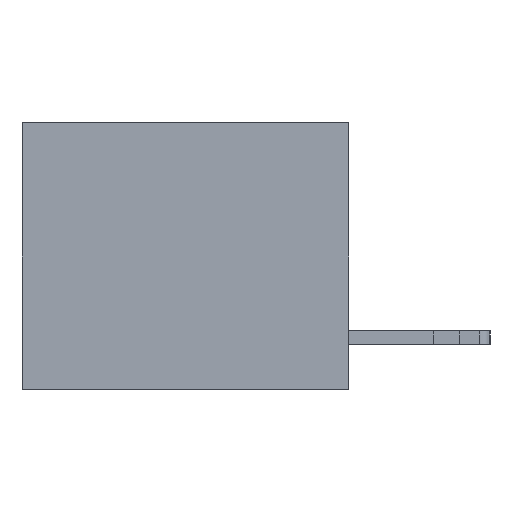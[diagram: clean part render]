
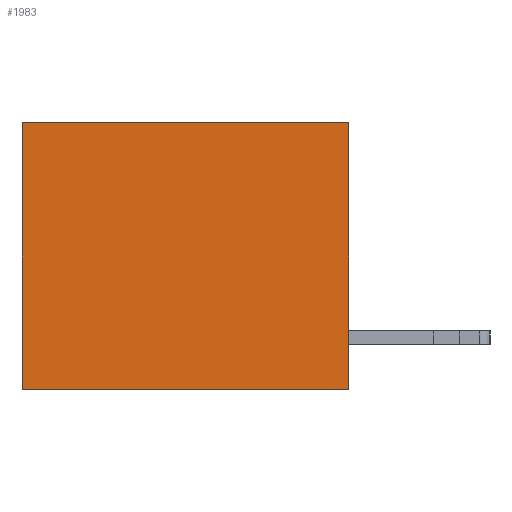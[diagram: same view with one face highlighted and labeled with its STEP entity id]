
A CAD part, left-side view. The second image highlights one B-rep face of the part: STEP entity #1983.
In plain terms, the highlighted planar face has unit normal (-1, 0, 0).
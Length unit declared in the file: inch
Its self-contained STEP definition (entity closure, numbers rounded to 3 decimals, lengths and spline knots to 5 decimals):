
#357 = EDGE_CURVE ( 'NONE', #7541, #11185, #21922, .T. ) ;
#1149 = DIRECTION ( 'NONE',  ( 0., 0., -1. ) ) ;
#1983 = ADVANCED_FACE ( 'NONE', ( #4147 ), #3346, .F. ) ;
#2120 = VECTOR ( 'NONE', #2600, 39.37008 ) ;
#2600 = DIRECTION ( 'NONE',  ( 0., 1., 0. ) ) ;
#2934 = EDGE_CURVE ( 'NONE', #11185, #13010, #17881, .T. ) ;
#3230 = DIRECTION ( 'NONE',  ( 0., 1., 0. ) ) ;
#3346 = PLANE ( 'NONE',  #8879 ) ;
#4147 = FACE_OUTER_BOUND ( 'NONE', #4402, .T. ) ;
#4402 = EDGE_LOOP ( 'NONE', ( #14719, #14878, #11434, #5678 ) ) ;
#4917 = CARTESIAN_POINT ( 'NONE',  ( 0.3165, 0.6, -0.49 ) ) ;
#5678 = ORIENTED_EDGE ( 'NONE', *, *, #357, .T. ) ;
#5765 = EDGE_CURVE ( 'NONE', #7255, #13010, #18853, .T. ) ;
#5997 = EDGE_CURVE ( 'NONE', #7541, #7255, #20634, .T. ) ;
#6631 = CARTESIAN_POINT ( 'NONE',  ( 0.3165, 0., -0.49 ) ) ;
#7255 = VERTEX_POINT ( 'NONE', #9803 ) ;
#7541 = VERTEX_POINT ( 'NONE', #13903 ) ;
#7947 = CARTESIAN_POINT ( 'NONE',  ( 0.3165, 0., -0.49 ) ) ;
#8518 = VECTOR ( 'NONE', #1149, 39.37008 ) ;
#8879 = AXIS2_PLACEMENT_3D ( 'NONE', #10184, #21768, #20356 ) ;
#9803 = CARTESIAN_POINT ( 'NONE',  ( 0.3165, 0., -0.49 ) ) ;
#10184 = CARTESIAN_POINT ( 'NONE',  ( 0.3165, 0., -0.49 ) ) ;
#11185 = VERTEX_POINT ( 'NONE', #17827 ) ;
#11434 = ORIENTED_EDGE ( 'NONE', *, *, #5997, .F. ) ;
#13010 = VERTEX_POINT ( 'NONE', #20345 ) ;
#13903 = CARTESIAN_POINT ( 'NONE',  ( 0.3165, 0., 0. ) ) ;
#14164 = VECTOR ( 'NONE', #16894, 39.37008 ) ;
#14719 = ORIENTED_EDGE ( 'NONE', *, *, #2934, .T. ) ;
#14878 = ORIENTED_EDGE ( 'NONE', *, *, #5765, .F. ) ;
#15597 = VECTOR ( 'NONE', #3230, 39.37008 ) ;
#16894 = DIRECTION ( 'NONE',  ( 0., 0., -1. ) ) ;
#17827 = CARTESIAN_POINT ( 'NONE',  ( 0.3165, 0.6, 0. ) ) ;
#17881 = LINE ( 'NONE', #4917, #14164 ) ;
#18853 = LINE ( 'NONE', #6631, #2120 ) ;
#19637 = CARTESIAN_POINT ( 'NONE',  ( 0.3165, 0., 0. ) ) ;
#20345 = CARTESIAN_POINT ( 'NONE',  ( 0.3165, 0.6, -0.49 ) ) ;
#20356 = DIRECTION ( 'NONE',  ( 0., 0., -1. ) ) ;
#20634 = LINE ( 'NONE', #7947, #8518 ) ;
#21768 = DIRECTION ( 'NONE',  ( 1., 0., 0. ) ) ;
#21922 = LINE ( 'NONE', #19637, #15597 ) ;
